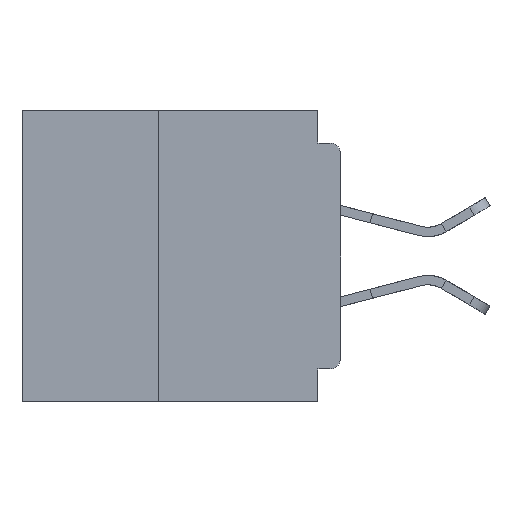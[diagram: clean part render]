
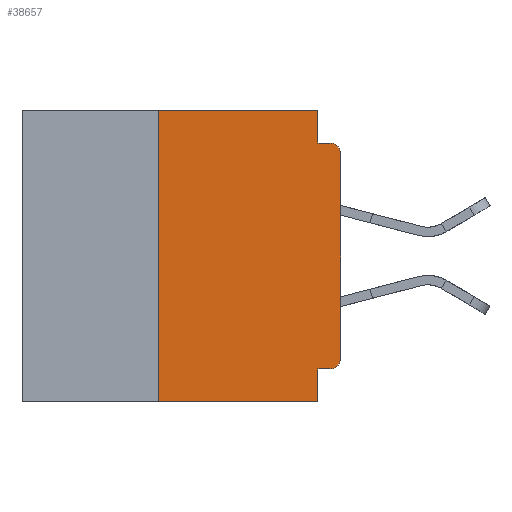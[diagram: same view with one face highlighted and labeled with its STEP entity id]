
A CAD part, left-side view. The second image highlights one B-rep face of the part: STEP entity #38657.
In plain terms, the highlighted planar face has unit normal (-1, 0, 0).
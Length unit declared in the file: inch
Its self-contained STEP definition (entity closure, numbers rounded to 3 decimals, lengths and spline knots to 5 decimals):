
#533 = VERTEX_POINT ( 'NONE', #18690 ) ;
#593 = AXIS2_PLACEMENT_3D ( 'NONE', #22332, #12958, #34943 ) ;
#1075 = ORIENTED_EDGE ( 'NONE', *, *, #10778, .F. ) ;
#1085 = ORIENTED_EDGE ( 'NONE', *, *, #37141, .T. ) ;
#1680 = CARTESIAN_POINT ( 'NONE',  ( 0., 0.031, 0. ) ) ;
#1740 = LINE ( 'NONE', #33664, #34365 ) ;
#1893 = ORIENTED_EDGE ( 'NONE', *, *, #39908, .T. ) ;
#2079 = DIRECTION ( 'NONE',  ( 0., 0., -1. ) ) ;
#2162 = DIRECTION ( 'NONE',  ( 0., 0., -1. ) ) ;
#2982 = EDGE_CURVE ( 'NONE', #6812, #38342, #8429, .T. ) ;
#3239 = CARTESIAN_POINT ( 'NONE',  ( 0., 0.031, -0.4 ) ) ;
#3519 = CIRCLE ( 'NONE', #23908, 0.015 ) ;
#3640 = DIRECTION ( 'NONE',  ( 0., -1., 0. ) ) ;
#4156 = ORIENTED_EDGE ( 'NONE', *, *, #13000, .F. ) ;
#4386 = LINE ( 'NONE', #3239, #27640 ) ;
#4618 = DIRECTION ( 'NONE',  ( 0., 1., 0. ) ) ;
#4778 = CARTESIAN_POINT ( 'NONE',  ( 0., 0.25, -0.4 ) ) ;
#5073 = VERTEX_POINT ( 'NONE', #12255 ) ;
#6563 = CARTESIAN_POINT ( 'NONE',  ( 0., 0.437, -0.4 ) ) ;
#6692 = DIRECTION ( 'NONE',  ( 0., -1., 0. ) ) ;
#6812 = VERTEX_POINT ( 'NONE', #4778 ) ;
#7361 = LINE ( 'NONE', #14911, #31557 ) ;
#8429 = LINE ( 'NONE', #6563, #32585 ) ;
#8613 = DIRECTION ( 'NONE',  ( 0., 0., 1. ) ) ;
#9399 = LINE ( 'NONE', #13592, #25181 ) ;
#10166 = VECTOR ( 'NONE', #8613, 39.37008 ) ;
#10778 = EDGE_CURVE ( 'NONE', #28112, #38342, #4386, .T. ) ;
#10838 = EDGE_CURVE ( 'NONE', #32103, #30999, #25666, .T. ) ;
#10914 = CARTESIAN_POINT ( 'NONE',  ( 0., 0.25, 0. ) ) ;
#11275 = VERTEX_POINT ( 'NONE', #18264 ) ;
#11760 = EDGE_CURVE ( 'NONE', #36342, #5073, #7361, .T. ) ;
#12255 = CARTESIAN_POINT ( 'NONE',  ( 0., 0.015, -0.045 ) ) ;
#12652 = VERTEX_POINT ( 'NONE', #38194 ) ;
#12932 = VECTOR ( 'NONE', #4618, 39.37008 ) ;
#12958 = DIRECTION ( 'NONE',  ( 1., 0., 0. ) ) ;
#13000 = EDGE_CURVE ( 'NONE', #30999, #36342, #1740, .T. ) ;
#13592 = CARTESIAN_POINT ( 'NONE',  ( 0., 0., 0. ) ) ;
#14911 = CARTESIAN_POINT ( 'NONE',  ( 0., 0., -0.045 ) ) ;
#15857 = DIRECTION ( 'NONE',  ( 0., 0., -1. ) ) ;
#17041 = EDGE_CURVE ( 'NONE', #6812, #32103, #17549, .T. ) ;
#17549 = LINE ( 'NONE', #18002, #10166 ) ;
#17621 = DIRECTION ( 'NONE',  ( -1., 0., 0. ) ) ;
#18002 = CARTESIAN_POINT ( 'NONE',  ( 0., 0.25, -0.4 ) ) ;
#18264 = CARTESIAN_POINT ( 'NONE',  ( 0., 0.015, -0.355 ) ) ;
#18690 = CARTESIAN_POINT ( 'NONE',  ( 0., 0., -0.06 ) ) ;
#19418 = CARTESIAN_POINT ( 'NONE',  ( 0., 0.437, 0. ) ) ;
#20038 = CARTESIAN_POINT ( 'NONE',  ( 0., 0.031, -0.045 ) ) ;
#20974 = EDGE_CURVE ( 'NONE', #12652, #533, #9399, .T. ) ;
#21040 = DIRECTION ( 'NONE',  ( -1., 0., 0. ) ) ;
#21870 = ORIENTED_EDGE ( 'NONE', *, *, #10838, .F. ) ;
#22308 = LINE ( 'NONE', #26747, #12932 ) ;
#22332 = CARTESIAN_POINT ( 'NONE',  ( 0., 0.437, 0. ) ) ;
#23908 = AXIS2_PLACEMENT_3D ( 'NONE', #39871, #21040, #2079 ) ;
#23957 = ORIENTED_EDGE ( 'NONE', *, *, #20974, .T. ) ;
#24210 = ORIENTED_EDGE ( 'NONE', *, *, #28100, .F. ) ;
#25181 = VECTOR ( 'NONE', #35585, 39.37008 ) ;
#25504 = PLANE ( 'NONE',  #593 ) ;
#25666 = LINE ( 'NONE', #19418, #33017 ) ;
#26747 = CARTESIAN_POINT ( 'NONE',  ( 0., 0., -0.355 ) ) ;
#26880 = CARTESIAN_POINT ( 'NONE',  ( 0., 0.031, -0.355 ) ) ;
#27640 = VECTOR ( 'NONE', #15857, 39.37008 ) ;
#28100 = EDGE_CURVE ( 'NONE', #11275, #28112, #22308, .T. ) ;
#28112 = VERTEX_POINT ( 'NONE', #26880 ) ;
#28556 = ORIENTED_EDGE ( 'NONE', *, *, #2982, .T. ) ;
#29358 = ORIENTED_EDGE ( 'NONE', *, *, #11760, .F. ) ;
#30198 = CARTESIAN_POINT ( 'NONE',  ( 0., 0.031, -0.4 ) ) ;
#30546 = AXIS2_PLACEMENT_3D ( 'NONE', #36432, #17621, #39609 ) ;
#30809 = EDGE_LOOP ( 'NONE', ( #23957, #1085, #29358, #4156, #21870, #36465, #28556, #1075, #24210, #1893 ) ) ;
#30999 = VERTEX_POINT ( 'NONE', #1680 ) ;
#31557 = VECTOR ( 'NONE', #40059, 39.37008 ) ;
#32103 = VERTEX_POINT ( 'NONE', #10914 ) ;
#32585 = VECTOR ( 'NONE', #6692, 39.37008 ) ;
#33017 = VECTOR ( 'NONE', #3640, 39.37008 ) ;
#33664 = CARTESIAN_POINT ( 'NONE',  ( 0., 0.031, 0. ) ) ;
#34365 = VECTOR ( 'NONE', #2162, 39.37008 ) ;
#34943 = DIRECTION ( 'NONE',  ( 0., 0., -1. ) ) ;
#35428 = FACE_OUTER_BOUND ( 'NONE', #30809, .T. ) ;
#35585 = DIRECTION ( 'NONE',  ( 0., 0., 1. ) ) ;
#36283 = CIRCLE ( 'NONE', #30546, 0.015 ) ;
#36342 = VERTEX_POINT ( 'NONE', #20038 ) ;
#36432 = CARTESIAN_POINT ( 'NONE',  ( 0., 0.015, -0.34 ) ) ;
#36465 = ORIENTED_EDGE ( 'NONE', *, *, #17041, .F. ) ;
#37141 = EDGE_CURVE ( 'NONE', #533, #5073, #3519, .T. ) ;
#38194 = CARTESIAN_POINT ( 'NONE',  ( 0., 0., -0.34 ) ) ;
#38342 = VERTEX_POINT ( 'NONE', #30198 ) ;
#38657 = ADVANCED_FACE ( 'NONE', ( #35428 ), #25504, .F. ) ;
#39609 = DIRECTION ( 'NONE',  ( 0., 0., -1. ) ) ;
#39871 = CARTESIAN_POINT ( 'NONE',  ( 0., 0.015, -0.06 ) ) ;
#39908 = EDGE_CURVE ( 'NONE', #11275, #12652, #36283, .T. ) ;
#40059 = DIRECTION ( 'NONE',  ( 0., -1., 0. ) ) ;
